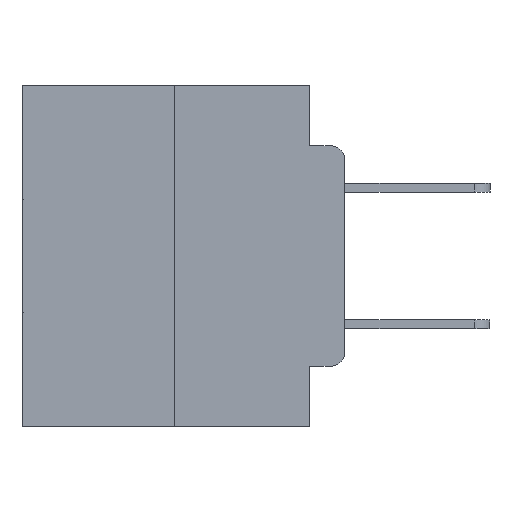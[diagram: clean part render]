
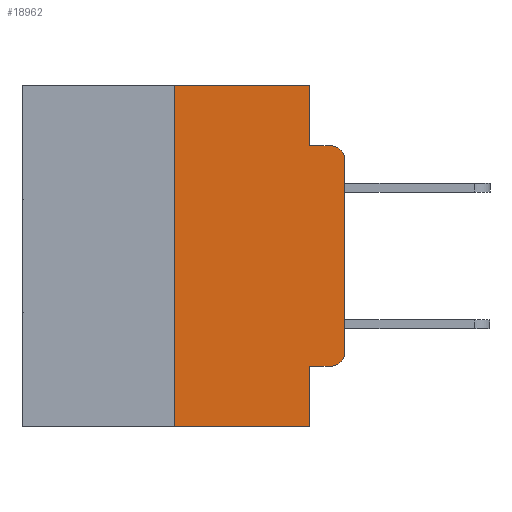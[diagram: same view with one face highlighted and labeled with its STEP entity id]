
A CAD part, left-side view. The second image highlights one B-rep face of the part: STEP entity #18962.
In plain terms, the highlighted planar face has unit normal (-1, 0, 0).
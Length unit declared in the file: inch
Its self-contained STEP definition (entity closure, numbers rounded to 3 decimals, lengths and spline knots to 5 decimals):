
#67 = VERTEX_POINT ( 'NONE', #12365 ) ;
#909 = DIRECTION ( 'NONE',  ( 0., 0., -1. ) ) ;
#1146 = ORIENTED_EDGE ( 'NONE', *, *, #23763, .F. ) ;
#1340 = CARTESIAN_POINT ( 'NONE',  ( 0., 0.051, -0.4115 ) ) ;
#1667 = CARTESIAN_POINT ( 'NONE',  ( 0., 0.473, 0. ) ) ;
#2356 = DIRECTION ( 'NONE',  ( 0., -1., 0. ) ) ;
#2696 = CARTESIAN_POINT ( 'NONE',  ( 0., 0., 0. ) ) ;
#3090 = EDGE_CURVE ( 'NONE', #10376, #17518, #3098, .T. ) ;
#3098 = CIRCLE ( 'NONE', #4977, 0.02 ) ;
#3152 = CARTESIAN_POINT ( 'NONE',  ( 0., 0., -0.3915 ) ) ;
#3155 = LINE ( 'NONE', #9694, #25229 ) ;
#3919 = ORIENTED_EDGE ( 'NONE', *, *, #19522, .T. ) ;
#4018 = DIRECTION ( 'NONE',  ( -1., 0., 0. ) ) ;
#4977 = AXIS2_PLACEMENT_3D ( 'NONE', #19308, #6412, #7835 ) ;
#5495 = DIRECTION ( 'NONE',  ( 0., 0., 1. ) ) ;
#5496 = VECTOR ( 'NONE', #12556, 39.37008 ) ;
#5516 = VECTOR ( 'NONE', #2356, 39.37008 ) ;
#6412 = DIRECTION ( 'NONE',  ( -1., 0., 0. ) ) ;
#7177 = CARTESIAN_POINT ( 'NONE',  ( 0., 0.473, -0.5 ) ) ;
#7447 = VECTOR ( 'NONE', #25020, 39.37008 ) ;
#7564 = VERTEX_POINT ( 'NONE', #20490 ) ;
#7835 = DIRECTION ( 'NONE',  ( 0., 0., -1. ) ) ;
#8265 = ORIENTED_EDGE ( 'NONE', *, *, #20959, .F. ) ;
#8392 = VERTEX_POINT ( 'NONE', #18954 ) ;
#8945 = ORIENTED_EDGE ( 'NONE', *, *, #22407, .T. ) ;
#9181 = VECTOR ( 'NONE', #13405, 39.37008 ) ;
#9195 = EDGE_CURVE ( 'NONE', #20052, #67, #9867, .T. ) ;
#9264 = ORIENTED_EDGE ( 'NONE', *, *, #17319, .T. ) ;
#9548 = AXIS2_PLACEMENT_3D ( 'NONE', #16856, #4018, #19074 ) ;
#9694 = CARTESIAN_POINT ( 'NONE',  ( 0., 0.25, 0. ) ) ;
#9867 = LINE ( 'NONE', #17395, #5516 ) ;
#10312 = EDGE_CURVE ( 'NONE', #18506, #17518, #16892, .T. ) ;
#10315 = VECTOR ( 'NONE', #18698, 39.37008 ) ;
#10329 = DIRECTION ( 'NONE',  ( 0., 0., -1. ) ) ;
#10376 = VERTEX_POINT ( 'NONE', #19249 ) ;
#10622 = ORIENTED_EDGE ( 'NONE', *, *, #10312, .F. ) ;
#11670 = LINE ( 'NONE', #1340, #10315 ) ;
#11804 = VERTEX_POINT ( 'NONE', #17770 ) ;
#11975 = ORIENTED_EDGE ( 'NONE', *, *, #9195, .F. ) ;
#12365 = CARTESIAN_POINT ( 'NONE',  ( 0., 0.051, 0. ) ) ;
#12556 = DIRECTION ( 'NONE',  ( 0., -1., 0. ) ) ;
#12643 = ORIENTED_EDGE ( 'NONE', *, *, #12987, .T. ) ;
#12987 = EDGE_CURVE ( 'NONE', #8392, #7564, #26634, .T. ) ;
#13160 = LINE ( 'NONE', #16475, #7447 ) ;
#13405 = DIRECTION ( 'NONE',  ( 0., 0., 1. ) ) ;
#13774 = FACE_OUTER_BOUND ( 'NONE', #15427, .T. ) ;
#13991 = LINE ( 'NONE', #24133, #24428 ) ;
#14207 = LINE ( 'NONE', #2696, #9181 ) ;
#15427 = EDGE_LOOP ( 'NONE', ( #9264, #20732, #10622, #22085, #11975, #1146, #12643, #8265, #8945, #3919 ) ) ;
#16475 = CARTESIAN_POINT ( 'NONE',  ( 0., 0.051, 0. ) ) ;
#16856 = CARTESIAN_POINT ( 'NONE',  ( 0., 0.02, -0.3915 ) ) ;
#16892 = LINE ( 'NONE', #23233, #5496 ) ;
#17319 = EDGE_CURVE ( 'NONE', #24969, #10376, #14207, .T. ) ;
#17395 = CARTESIAN_POINT ( 'NONE',  ( 0., 0.473, 0. ) ) ;
#17518 = VERTEX_POINT ( 'NONE', #22708 ) ;
#17770 = CARTESIAN_POINT ( 'NONE',  ( 0., 0.051, -0.4115 ) ) ;
#17866 = AXIS2_PLACEMENT_3D ( 'NONE', #1667, #23174, #10329 ) ;
#18506 = VERTEX_POINT ( 'NONE', #19498 ) ;
#18698 = DIRECTION ( 'NONE',  ( 0., -1., 0. ) ) ;
#18717 = CARTESIAN_POINT ( 'NONE',  ( 0., 0.02, -0.4115 ) ) ;
#18954 = CARTESIAN_POINT ( 'NONE',  ( 0., 0.25, -0.5 ) ) ;
#18962 = ADVANCED_FACE ( 'NONE', ( #13774 ), #23095, .F. ) ;
#19074 = DIRECTION ( 'NONE',  ( 0., 0., -1. ) ) ;
#19249 = CARTESIAN_POINT ( 'NONE',  ( 0., 0., -0.1085 ) ) ;
#19308 = CARTESIAN_POINT ( 'NONE',  ( 0., 0.02, -0.1085 ) ) ;
#19498 = CARTESIAN_POINT ( 'NONE',  ( 0., 0.051, -0.0885 ) ) ;
#19522 = EDGE_CURVE ( 'NONE', #24523, #24969, #27313, .T. ) ;
#20052 = VERTEX_POINT ( 'NONE', #26971 ) ;
#20066 = DIRECTION ( 'NONE',  ( 0., -1., 0. ) ) ;
#20490 = CARTESIAN_POINT ( 'NONE',  ( 0., 0.051, -0.5 ) ) ;
#20732 = ORIENTED_EDGE ( 'NONE', *, *, #3090, .T. ) ;
#20959 = EDGE_CURVE ( 'NONE', #11804, #7564, #13991, .T. ) ;
#22085 = ORIENTED_EDGE ( 'NONE', *, *, #25119, .F. ) ;
#22407 = EDGE_CURVE ( 'NONE', #11804, #24523, #11670, .T. ) ;
#22708 = CARTESIAN_POINT ( 'NONE',  ( 0., 0.02, -0.0885 ) ) ;
#23095 = PLANE ( 'NONE',  #17866 ) ;
#23174 = DIRECTION ( 'NONE',  ( 1., 0., 0. ) ) ;
#23233 = CARTESIAN_POINT ( 'NONE',  ( 0., 0.051, -0.0885 ) ) ;
#23763 = EDGE_CURVE ( 'NONE', #8392, #20052, #3155, .T. ) ;
#24133 = CARTESIAN_POINT ( 'NONE',  ( 0., 0.051, 0. ) ) ;
#24428 = VECTOR ( 'NONE', #909, 39.37008 ) ;
#24523 = VERTEX_POINT ( 'NONE', #18717 ) ;
#24969 = VERTEX_POINT ( 'NONE', #3152 ) ;
#25020 = DIRECTION ( 'NONE',  ( 0., 0., -1. ) ) ;
#25119 = EDGE_CURVE ( 'NONE', #67, #18506, #13160, .T. ) ;
#25229 = VECTOR ( 'NONE', #5495, 39.37008 ) ;
#26634 = LINE ( 'NONE', #7177, #27281 ) ;
#26971 = CARTESIAN_POINT ( 'NONE',  ( 0., 0.25, 0. ) ) ;
#27281 = VECTOR ( 'NONE', #20066, 39.37008 ) ;
#27313 = CIRCLE ( 'NONE', #9548, 0.02 ) ;
